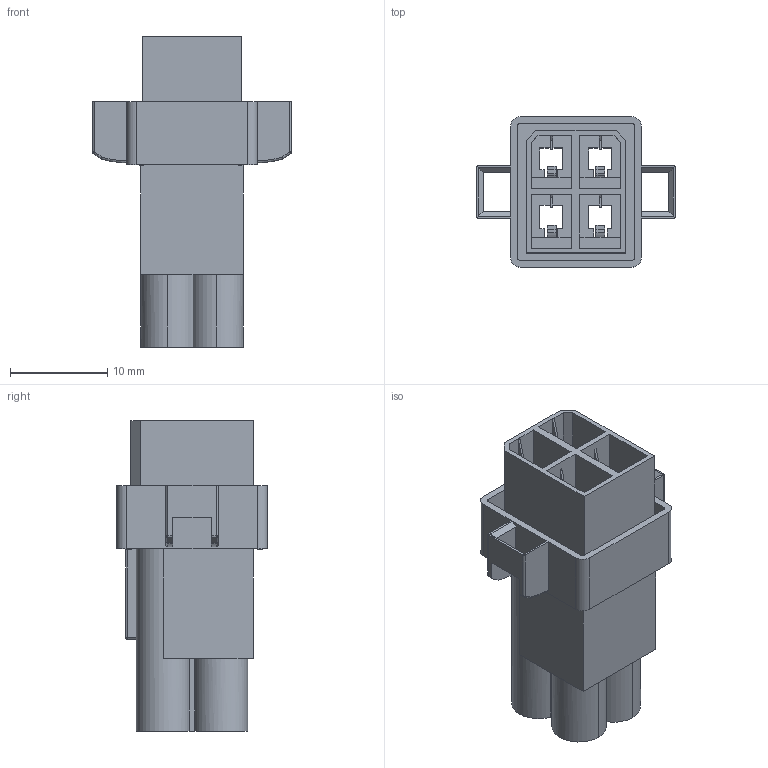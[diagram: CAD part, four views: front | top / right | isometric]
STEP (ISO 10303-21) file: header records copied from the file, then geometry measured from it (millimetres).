
FILE_DESCRIPTION (( 'STEP AP214' ), '1' );
FILE_NAME ('567-004-000-310.STEP', '2020-07-27T20:06:19', ( '' ), ( '' ), 'SwSTEP 2.0', 'SolidWorks 2020', '' );
FILE_SCHEMA (( 'AUTOMOTIVE_DESIGN' ));
Length unit declared in the file: millimetre
Products named in the file (1): 567-004-000-310
Bounding box: 20.5 x 15.5 x 32 mm (x, y, z)
Volume: 2039.6 mm3; surface area: 5052.9 mm2
Topology: 1 solids, 9 shells, 410 faces, 1109 edges, 718 vertices
Faces by surface type: plane 317, cylinder 59, bspline 20, sphere 10, torus 4
Entity records: 13781 total; most frequent: CARTESIAN_POINT 3494, ORIENTED_EDGE 2206, DIRECTION 1993, EDGE_CURVE 1103, VECTOR 887, LINE 887, VERTEX_POINT 718, AXIS2_PLACEMENT_3D 553
